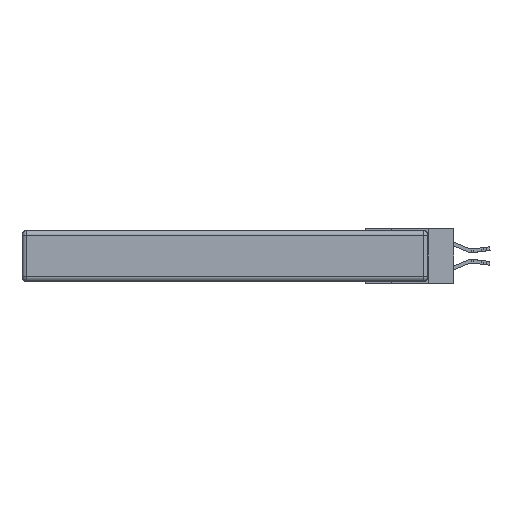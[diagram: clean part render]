
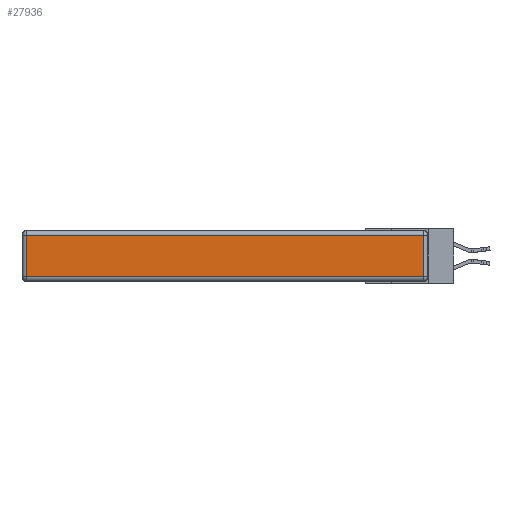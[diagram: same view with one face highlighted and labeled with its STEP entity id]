
A CAD part, left-side view. The second image highlights one B-rep face of the part: STEP entity #27936.
In plain terms, the highlighted planar face has unit normal (-1, 0, 0).
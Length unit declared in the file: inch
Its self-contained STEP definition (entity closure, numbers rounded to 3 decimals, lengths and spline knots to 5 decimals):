
#187 = LINE ( 'NONE', #9935, #4387 ) ;
#1255 = VERTEX_POINT ( 'NONE', #12260 ) ;
#1365 = VERTEX_POINT ( 'NONE', #11845 ) ;
#1850 = ORIENTED_EDGE ( 'NONE', *, *, #17232, .T. ) ;
#2188 = ORIENTED_EDGE ( 'NONE', *, *, #23835, .T. ) ;
#2994 = DIRECTION ( 'NONE',  ( 0., -1., 0. ) ) ;
#4105 = LINE ( 'NONE', #30764, #9754 ) ;
#4215 = VERTEX_POINT ( 'NONE', #22486 ) ;
#4387 = VECTOR ( 'NONE', #26589, 39.37008 ) ;
#5246 = LINE ( 'NONE', #28524, #17330 ) ;
#5483 = ORIENTED_EDGE ( 'NONE', *, *, #25423, .T. ) ;
#5715 = ORIENTED_EDGE ( 'NONE', *, *, #24119, .T. ) ;
#6578 = VERTEX_POINT ( 'NONE', #14758 ) ;
#7628 = EDGE_LOOP ( 'NONE', ( #5715, #2188, #1850, #5483 ) ) ;
#7769 = DIRECTION ( 'NONE',  ( 0., 0., 1. ) ) ;
#9640 = DIRECTION ( 'NONE',  ( 0., 1., 0. ) ) ;
#9754 = VECTOR ( 'NONE', #23634, 39.37008 ) ;
#9935 = CARTESIAN_POINT ( 'NONE',  ( 0., 2.72, -0.343 ) ) ;
#11771 = FACE_OUTER_BOUND ( 'NONE', #7628, .T. ) ;
#11845 = CARTESIAN_POINT ( 'NONE',  ( 0., 0.03, -0.03 ) ) ;
#12260 = CARTESIAN_POINT ( 'NONE',  ( 0., 2.72, -0.313 ) ) ;
#14758 = CARTESIAN_POINT ( 'NONE',  ( 0., 0.03, -0.313 ) ) ;
#14955 = AXIS2_PLACEMENT_3D ( 'NONE', #22248, #17301, #7769 ) ;
#17232 = EDGE_CURVE ( 'NONE', #1365, #4215, #5246, .T. ) ;
#17301 = DIRECTION ( 'NONE',  ( -1., 0., 0. ) ) ;
#17330 = VECTOR ( 'NONE', #9640, 39.37008 ) ;
#19596 = VECTOR ( 'NONE', #2994, 39.37008 ) ;
#22035 = PLANE ( 'NONE',  #14955 ) ;
#22248 = CARTESIAN_POINT ( 'NONE',  ( 0., 0., -0.343 ) ) ;
#22336 = CARTESIAN_POINT ( 'NONE',  ( 0., 0., -0.313 ) ) ;
#22486 = CARTESIAN_POINT ( 'NONE',  ( 0., 2.72, -0.03 ) ) ;
#23634 = DIRECTION ( 'NONE',  ( 0., 0., 1. ) ) ;
#23835 = EDGE_CURVE ( 'NONE', #6578, #1365, #4105, .T. ) ;
#24119 = EDGE_CURVE ( 'NONE', #1255, #6578, #25972, .T. ) ;
#25423 = EDGE_CURVE ( 'NONE', #4215, #1255, #187, .T. ) ;
#25972 = LINE ( 'NONE', #22336, #19596 ) ;
#26589 = DIRECTION ( 'NONE',  ( 0., 0., -1. ) ) ;
#27936 = ADVANCED_FACE ( 'NONE', ( #11771 ), #22035, .T. ) ;
#28524 = CARTESIAN_POINT ( 'NONE',  ( 0., 2.75, -0.03 ) ) ;
#30764 = CARTESIAN_POINT ( 'NONE',  ( 0., 0.03, -0.343 ) ) ;
